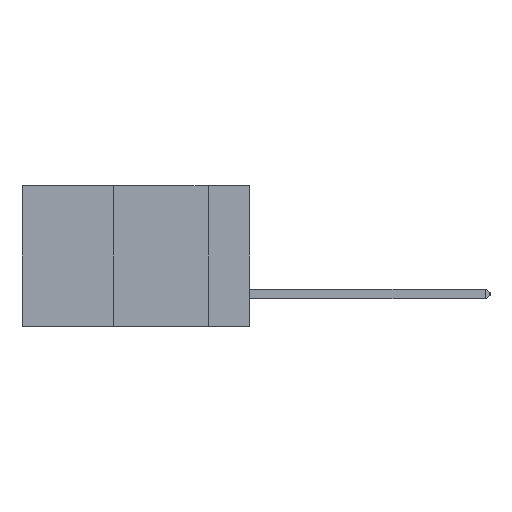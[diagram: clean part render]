
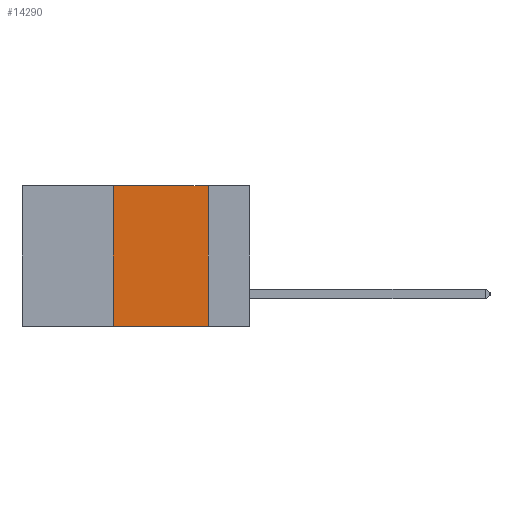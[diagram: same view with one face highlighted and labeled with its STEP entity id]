
A CAD part, left-side view. The second image highlights one B-rep face of the part: STEP entity #14290.
In plain terms, the highlighted planar face has unit normal (-1, 0, 0).
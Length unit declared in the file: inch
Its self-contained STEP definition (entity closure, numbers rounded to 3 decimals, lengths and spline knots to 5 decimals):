
#74 = ORIENTED_EDGE ( 'NONE', *, *, #21569, .F. ) ;
#370 = DIRECTION ( 'NONE',  ( 0., -1., 0. ) ) ;
#1252 = EDGE_CURVE ( 'NONE', #17461, #6766, #14643, .T. ) ;
#1674 = DIRECTION ( 'NONE',  ( 0., -1., 0. ) ) ;
#3577 = ORIENTED_EDGE ( 'NONE', *, *, #5018, .F. ) ;
#4555 = CARTESIAN_POINT ( 'NONE',  ( 0., 0.11, 0. ) ) ;
#4878 = LINE ( 'NONE', #10461, #10404 ) ;
#4889 = VECTOR ( 'NONE', #1674, 39.37008 ) ;
#5018 = EDGE_CURVE ( 'NONE', #17461, #5534, #12906, .T. ) ;
#5337 = CARTESIAN_POINT ( 'NONE',  ( 0., 0.6, 0. ) ) ;
#5534 = VERTEX_POINT ( 'NONE', #20051 ) ;
#5923 = FACE_OUTER_BOUND ( 'NONE', #8209, .T. ) ;
#6076 = VECTOR ( 'NONE', #6248, 39.37008 ) ;
#6248 = DIRECTION ( 'NONE',  ( 0., 0., -1. ) ) ;
#6766 = VERTEX_POINT ( 'NONE', #8046 ) ;
#8046 = CARTESIAN_POINT ( 'NONE',  ( 0., 0.11, -0.37 ) ) ;
#8209 = EDGE_LOOP ( 'NONE', ( #13688, #74, #3577, #20912 ) ) ;
#8772 = CARTESIAN_POINT ( 'NONE',  ( 0., 0.11, 0. ) ) ;
#9327 = DIRECTION ( 'NONE',  ( 0., 0., 1. ) ) ;
#9480 = VECTOR ( 'NONE', #9327, 39.37008 ) ;
#10118 = DIRECTION ( 'NONE',  ( 1., 0., 0. ) ) ;
#10227 = AXIS2_PLACEMENT_3D ( 'NONE', #5337, #10118, #20540 ) ;
#10404 = VECTOR ( 'NONE', #370, 39.37008 ) ;
#10461 = CARTESIAN_POINT ( 'NONE',  ( 0., 0.6, 0. ) ) ;
#12057 = EDGE_CURVE ( 'NONE', #19713, #6766, #16882, .T. ) ;
#12906 = LINE ( 'NONE', #19613, #9480 ) ;
#13562 = CARTESIAN_POINT ( 'NONE',  ( 0., 0.36, -0.37 ) ) ;
#13688 = ORIENTED_EDGE ( 'NONE', *, *, #12057, .F. ) ;
#14290 = ADVANCED_FACE ( 'NONE', ( #5923 ), #16910, .F. ) ;
#14643 = LINE ( 'NONE', #20477, #4889 ) ;
#16882 = LINE ( 'NONE', #4555, #6076 ) ;
#16910 = PLANE ( 'NONE',  #10227 ) ;
#17461 = VERTEX_POINT ( 'NONE', #13562 ) ;
#19613 = CARTESIAN_POINT ( 'NONE',  ( 0., 0.36, 0. ) ) ;
#19713 = VERTEX_POINT ( 'NONE', #8772 ) ;
#20051 = CARTESIAN_POINT ( 'NONE',  ( 0., 0.36, 0. ) ) ;
#20477 = CARTESIAN_POINT ( 'NONE',  ( 0., 0.6, -0.37 ) ) ;
#20540 = DIRECTION ( 'NONE',  ( 0., 0., -1. ) ) ;
#20912 = ORIENTED_EDGE ( 'NONE', *, *, #1252, .T. ) ;
#21569 = EDGE_CURVE ( 'NONE', #5534, #19713, #4878, .T. ) ;
